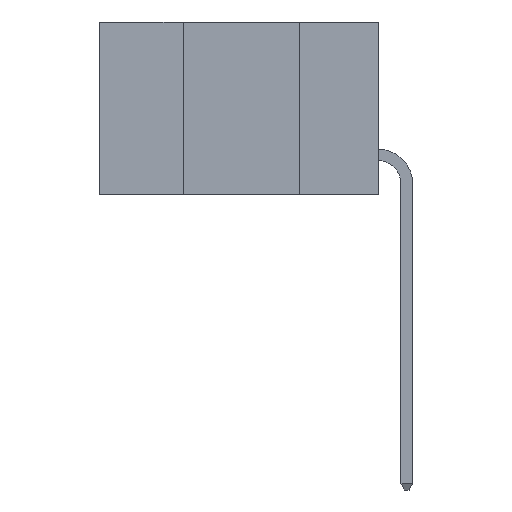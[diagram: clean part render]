
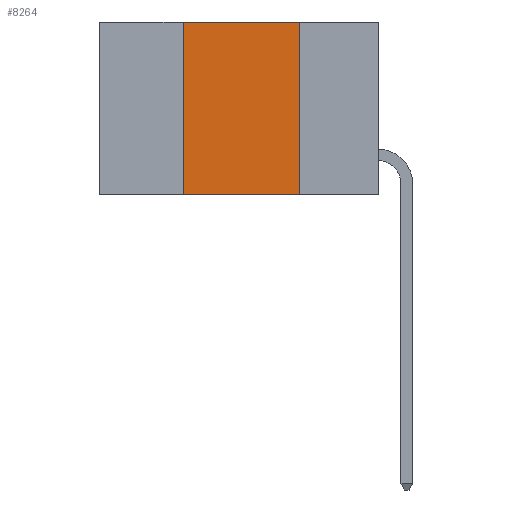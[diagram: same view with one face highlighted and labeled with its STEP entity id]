
A CAD part, left-side view. The second image highlights one B-rep face of the part: STEP entity #8264.
In plain terms, the highlighted planar face has unit normal (-1, 0, 0).
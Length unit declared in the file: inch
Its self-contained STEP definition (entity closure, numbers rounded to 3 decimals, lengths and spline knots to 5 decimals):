
#189 = LINE ( 'NONE', #17196, #19876 ) ;
#1826 = VERTEX_POINT ( 'NONE', #6293 ) ;
#2174 = VERTEX_POINT ( 'NONE', #15546 ) ;
#2612 = DIRECTION ( 'NONE',  ( 0., 0., 1. ) ) ;
#4588 = EDGE_CURVE ( 'NONE', #2174, #12220, #13519, .T. ) ;
#4705 = CARTESIAN_POINT ( 'NONE',  ( 0., 0.17, 0. ) ) ;
#4818 = VERTEX_POINT ( 'NONE', #5422 ) ;
#5422 = CARTESIAN_POINT ( 'NONE',  ( 0., 0.42, -0.37 ) ) ;
#5613 = EDGE_CURVE ( 'NONE', #4818, #1826, #13703, .T. ) ;
#6293 = CARTESIAN_POINT ( 'NONE',  ( 0., 0.17, -0.37 ) ) ;
#6428 = VECTOR ( 'NONE', #11928, 39.37008 ) ;
#8264 = ADVANCED_FACE ( 'NONE', ( #18232 ), #18271, .F. ) ;
#8415 = EDGE_CURVE ( 'NONE', #12220, #1826, #189, .T. ) ;
#9127 = EDGE_LOOP ( 'NONE', ( #9222, #15030, #14041, #16256 ) ) ;
#9222 = ORIENTED_EDGE ( 'NONE', *, *, #8415, .F. ) ;
#10288 = VECTOR ( 'NONE', #2612, 39.37008 ) ;
#10438 = CARTESIAN_POINT ( 'NONE',  ( 0., 0.42, -0.37 ) ) ;
#11928 = DIRECTION ( 'NONE',  ( 0., -1., 0. ) ) ;
#12039 = CARTESIAN_POINT ( 'NONE',  ( 0., 0.6, -0.37 ) ) ;
#12220 = VERTEX_POINT ( 'NONE', #4705 ) ;
#13196 = DIRECTION ( 'NONE',  ( 0., -1., 0. ) ) ;
#13519 = LINE ( 'NONE', #13819, #16694 ) ;
#13703 = LINE ( 'NONE', #12039, #6428 ) ;
#13819 = CARTESIAN_POINT ( 'NONE',  ( 0., 0.6, 0. ) ) ;
#14041 = ORIENTED_EDGE ( 'NONE', *, *, #19297, .F. ) ;
#15030 = ORIENTED_EDGE ( 'NONE', *, *, #4588, .F. ) ;
#15546 = CARTESIAN_POINT ( 'NONE',  ( 0., 0.42, 0. ) ) ;
#16256 = ORIENTED_EDGE ( 'NONE', *, *, #5613, .T. ) ;
#16694 = VECTOR ( 'NONE', #13196, 39.37008 ) ;
#17196 = CARTESIAN_POINT ( 'NONE',  ( 0., 0.17, -0.37 ) ) ;
#17279 = DIRECTION ( 'NONE',  ( 0., 0., -1. ) ) ;
#17999 = LINE ( 'NONE', #10438, #10288 ) ;
#18173 = DIRECTION ( 'NONE',  ( 0., 0., -1. ) ) ;
#18189 = DIRECTION ( 'NONE',  ( 1., 0., 0. ) ) ;
#18232 = FACE_OUTER_BOUND ( 'NONE', #9127, .T. ) ;
#18249 = CARTESIAN_POINT ( 'NONE',  ( 0., 0.6, 0. ) ) ;
#18271 = PLANE ( 'NONE',  #19073 ) ;
#19073 = AXIS2_PLACEMENT_3D ( 'NONE', #18249, #18189, #18173 ) ;
#19297 = EDGE_CURVE ( 'NONE', #4818, #2174, #17999, .T. ) ;
#19876 = VECTOR ( 'NONE', #17279, 39.37008 ) ;
